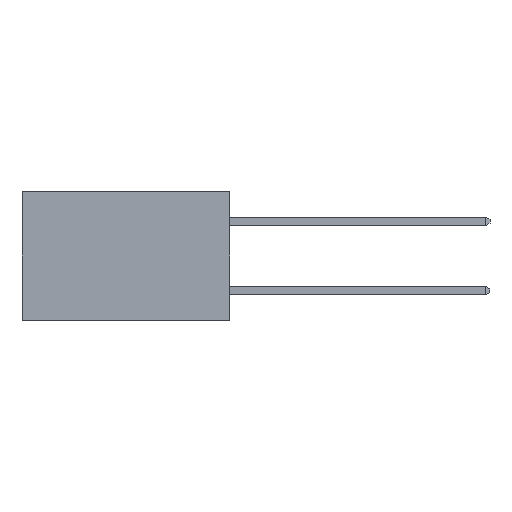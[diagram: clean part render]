
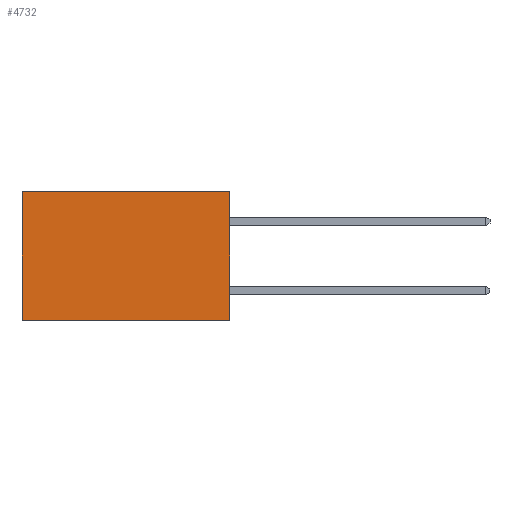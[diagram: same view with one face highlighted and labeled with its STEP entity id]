
A CAD part, left-side view. The second image highlights one B-rep face of the part: STEP entity #4732.
In plain terms, the highlighted planar face has unit normal (-1, 0, 0).
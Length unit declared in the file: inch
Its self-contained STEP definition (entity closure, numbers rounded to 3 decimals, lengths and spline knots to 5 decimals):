
#224 = LINE ( 'NONE', #5577, #3887 ) ;
#384 = FACE_OUTER_BOUND ( 'NONE', #1638, .T. ) ;
#452 = LINE ( 'NONE', #6193, #7626 ) ;
#650 = LINE ( 'NONE', #2124, #2512 ) ;
#696 = EDGE_CURVE ( 'NONE', #3107, #1215, #452, .T. ) ;
#953 = ORIENTED_EDGE ( 'NONE', *, *, #696, .T. ) ;
#1017 = DIRECTION ( 'NONE',  ( 0., 0., -1. ) ) ;
#1067 = DIRECTION ( 'NONE',  ( 1., 0., 0. ) ) ;
#1189 = DIRECTION ( 'NONE',  ( 0., 0., -1. ) ) ;
#1215 = VERTEX_POINT ( 'NONE', #1853 ) ;
#1431 = VERTEX_POINT ( 'NONE', #2665 ) ;
#1638 = EDGE_LOOP ( 'NONE', ( #953, #8735, #8855, #5232 ) ) ;
#1692 = CARTESIAN_POINT ( 'NONE',  ( 0.298, 0., 0. ) ) ;
#1853 = CARTESIAN_POINT ( 'NONE',  ( 0.298, 0.6, -0.37 ) ) ;
#1866 = CARTESIAN_POINT ( 'NONE',  ( 0.298, 0., -0.37 ) ) ;
#2124 = CARTESIAN_POINT ( 'NONE',  ( 0.298, 0., 0. ) ) ;
#2344 = EDGE_CURVE ( 'NONE', #1431, #3921, #7977, .T. ) ;
#2512 = VECTOR ( 'NONE', #2843, 39.37008 ) ;
#2621 = PLANE ( 'NONE',  #8247 ) ;
#2665 = CARTESIAN_POINT ( 'NONE',  ( 0.298, 0., 0. ) ) ;
#2843 = DIRECTION ( 'NONE',  ( 0., 1., 0. ) ) ;
#3107 = VERTEX_POINT ( 'NONE', #4664 ) ;
#3843 = VECTOR ( 'NONE', #1189, 39.37008 ) ;
#3887 = VECTOR ( 'NONE', #6225, 39.37008 ) ;
#3921 = VERTEX_POINT ( 'NONE', #1866 ) ;
#4664 = CARTESIAN_POINT ( 'NONE',  ( 0.298, 0.6, 0. ) ) ;
#4732 = ADVANCED_FACE ( 'NONE', ( #384 ), #2621, .F. ) ;
#5232 = ORIENTED_EDGE ( 'NONE', *, *, #7730, .T. ) ;
#5577 = CARTESIAN_POINT ( 'NONE',  ( 0.298, 0., -0.37 ) ) ;
#6193 = CARTESIAN_POINT ( 'NONE',  ( 0.298, 0.6, 0. ) ) ;
#6225 = DIRECTION ( 'NONE',  ( 0., 1., 0. ) ) ;
#6512 = DIRECTION ( 'NONE',  ( 0., 0., -1. ) ) ;
#7263 = EDGE_CURVE ( 'NONE', #3921, #1215, #224, .T. ) ;
#7626 = VECTOR ( 'NONE', #1017, 39.37008 ) ;
#7730 = EDGE_CURVE ( 'NONE', #1431, #3107, #650, .T. ) ;
#7977 = LINE ( 'NONE', #8002, #3843 ) ;
#8002 = CARTESIAN_POINT ( 'NONE',  ( 0.298, 0., 0. ) ) ;
#8247 = AXIS2_PLACEMENT_3D ( 'NONE', #1692, #1067, #6512 ) ;
#8735 = ORIENTED_EDGE ( 'NONE', *, *, #7263, .F. ) ;
#8855 = ORIENTED_EDGE ( 'NONE', *, *, #2344, .F. ) ;
